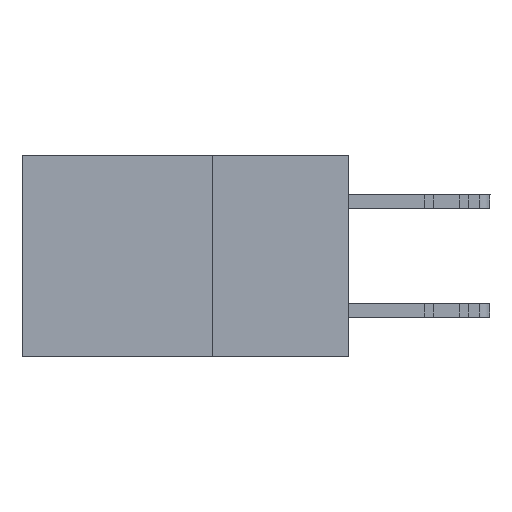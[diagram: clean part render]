
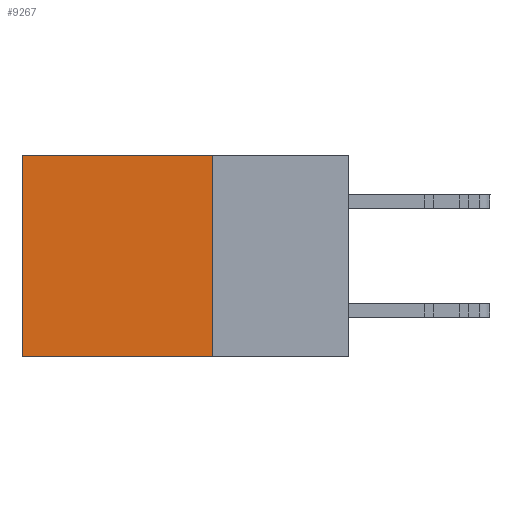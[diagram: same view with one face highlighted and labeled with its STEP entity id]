
A CAD part, left-side view. The second image highlights one B-rep face of the part: STEP entity #9267.
In plain terms, the highlighted planar face has unit normal (-1, 0, 0).
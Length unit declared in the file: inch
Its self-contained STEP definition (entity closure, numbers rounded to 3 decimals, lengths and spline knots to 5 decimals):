
#1160 = EDGE_CURVE ( 'NONE', #9149, #9742, #16576, .T. ) ;
#1253 = DIRECTION ( 'NONE',  ( 0., 0., -1. ) ) ;
#1645 = ORIENTED_EDGE ( 'NONE', *, *, #1160, .F. ) ;
#1823 = CARTESIAN_POINT ( 'NONE',  ( 0.298, 0.6, 0. ) ) ;
#2408 = AXIS2_PLACEMENT_3D ( 'NONE', #21698, #28391, #1253 ) ;
#3321 = LINE ( 'NONE', #17077, #26227 ) ;
#6282 = LINE ( 'NONE', #20053, #17729 ) ;
#6548 = EDGE_LOOP ( 'NONE', ( #28791, #1645, #18747, #14501 ) ) ;
#9149 = VERTEX_POINT ( 'NONE', #23201 ) ;
#9261 = LINE ( 'NONE', #16198, #18193 ) ;
#9267 = ADVANCED_FACE ( 'NONE', ( #12656 ), #10437, .F. ) ;
#9742 = VERTEX_POINT ( 'NONE', #24057 ) ;
#10224 = CARTESIAN_POINT ( 'NONE',  ( 0.298, 0.25, -0.37 ) ) ;
#10437 = PLANE ( 'NONE',  #2408 ) ;
#11541 = VECTOR ( 'NONE', #12725, 39.37008 ) ;
#12656 = FACE_OUTER_BOUND ( 'NONE', #6548, .T. ) ;
#12725 = DIRECTION ( 'NONE',  ( 0., 1., 0. ) ) ;
#14501 = ORIENTED_EDGE ( 'NONE', *, *, #15762, .T. ) ;
#15171 = DIRECTION ( 'NONE',  ( 0., 1., 0. ) ) ;
#15757 = VERTEX_POINT ( 'NONE', #1823 ) ;
#15762 = EDGE_CURVE ( 'NONE', #25106, #15757, #6282, .T. ) ;
#15913 = DIRECTION ( 'NONE',  ( 0., 0., -1. ) ) ;
#16198 = CARTESIAN_POINT ( 'NONE',  ( 0.298, 0.6, 0. ) ) ;
#16576 = LINE ( 'NONE', #10224, #11541 ) ;
#17077 = CARTESIAN_POINT ( 'NONE',  ( 0.298, 0.25, 0. ) ) ;
#17729 = VECTOR ( 'NONE', #15171, 39.37008 ) ;
#18193 = VECTOR ( 'NONE', #15913, 39.37008 ) ;
#18747 = ORIENTED_EDGE ( 'NONE', *, *, #23223, .F. ) ;
#20053 = CARTESIAN_POINT ( 'NONE',  ( 0.298, 0.25, 0. ) ) ;
#21698 = CARTESIAN_POINT ( 'NONE',  ( 0.298, 0.25, 0. ) ) ;
#23201 = CARTESIAN_POINT ( 'NONE',  ( 0.298, 0.25, -0.37 ) ) ;
#23223 = EDGE_CURVE ( 'NONE', #25106, #9149, #3321, .T. ) ;
#24057 = CARTESIAN_POINT ( 'NONE',  ( 0.298, 0.6, -0.37 ) ) ;
#24301 = EDGE_CURVE ( 'NONE', #15757, #9742, #9261, .T. ) ;
#25106 = VERTEX_POINT ( 'NONE', #28007 ) ;
#26144 = DIRECTION ( 'NONE',  ( 0., 0., -1. ) ) ;
#26227 = VECTOR ( 'NONE', #26144, 39.37008 ) ;
#28007 = CARTESIAN_POINT ( 'NONE',  ( 0.298, 0.25, 0. ) ) ;
#28391 = DIRECTION ( 'NONE',  ( 1., 0., 0. ) ) ;
#28791 = ORIENTED_EDGE ( 'NONE', *, *, #24301, .T. ) ;
